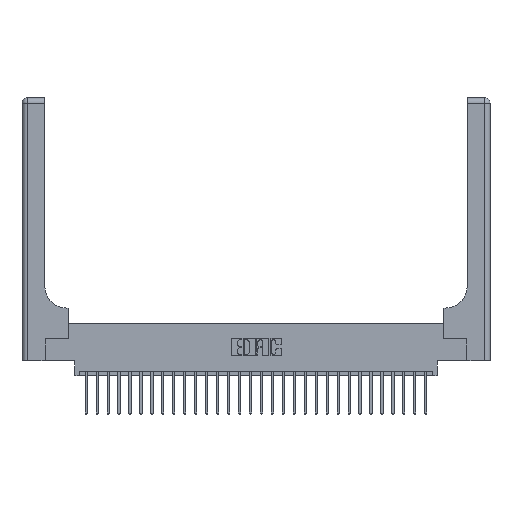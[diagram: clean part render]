
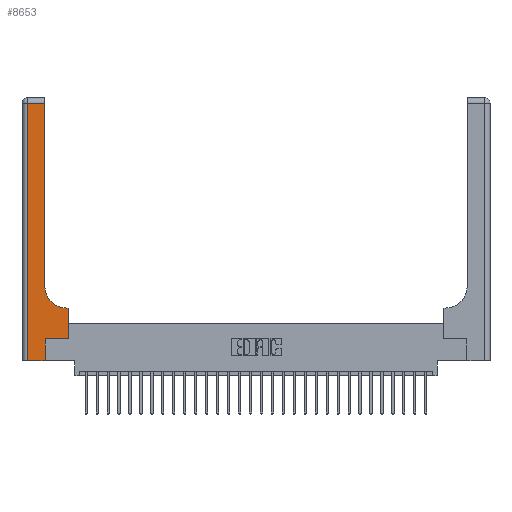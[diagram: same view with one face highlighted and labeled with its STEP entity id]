
A CAD part, top view. The second image highlights one B-rep face of the part: STEP entity #8653.
In plain terms, the highlighted planar face has unit normal (0, 0, 1).
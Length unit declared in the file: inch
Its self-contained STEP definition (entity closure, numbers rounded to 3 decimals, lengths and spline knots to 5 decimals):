
#243 = CARTESIAN_POINT ( 'NONE',  ( 0., 0., 0.37 ) ) ;
#2064 = VERTEX_POINT ( 'NONE', #19574 ) ;
#2099 = AXIS2_PLACEMENT_3D ( 'NONE', #23256, #10448, #25402 ) ;
#2349 = DIRECTION ( 'NONE',  ( 1., 0., 0. ) ) ;
#2496 = VERTEX_POINT ( 'NONE', #19162 ) ;
#2763 = EDGE_CURVE ( 'NONE', #27196, #2496, #19982, .T. ) ;
#3000 = VERTEX_POINT ( 'NONE', #27506 ) ;
#3001 = CIRCLE ( 'NONE', #2099, 0.25 ) ;
#3033 = LINE ( 'NONE', #22106, #20047 ) ;
#3495 = CARTESIAN_POINT ( 'NONE',  ( 0., 2.94, 0.37 ) ) ;
#3851 = VECTOR ( 'NONE', #6692, 39.37008 ) ;
#4194 = EDGE_CURVE ( 'NONE', #2064, #27196, #26249, .T. ) ;
#4537 = CARTESIAN_POINT ( 'NONE',  ( 0.528, 0.25, 0.37 ) ) ;
#4906 = CARTESIAN_POINT ( 'NONE',  ( 0.06, 2.94, 0.37 ) ) ;
#5364 = ORIENTED_EDGE ( 'NONE', *, *, #2763, .T. ) ;
#6692 = DIRECTION ( 'NONE',  ( 0., 1., 0. ) ) ;
#7667 = DIRECTION ( 'NONE',  ( 0., -1., 0. ) ) ;
#7842 = CARTESIAN_POINT ( 'NONE',  ( 0.26, 0.85, 0.37 ) ) ;
#8341 = VECTOR ( 'NONE', #26513, 39.37008 ) ;
#8450 = AXIS2_PLACEMENT_3D ( 'NONE', #23636, #10837, #25774 ) ;
#8653 = ADVANCED_FACE ( 'NONE', ( #12658 ), #19362, .F. ) ;
#8749 = CARTESIAN_POINT ( 'NONE',  ( 0.51, 0.6, 0.37 ) ) ;
#8845 = VECTOR ( 'NONE', #15403, 39.37008 ) ;
#8853 = EDGE_CURVE ( 'NONE', #15302, #2064, #12974, .T. ) ;
#9076 = EDGE_LOOP ( 'NONE', ( #20608, #18753, #5364, #17082, #13616, #17212, #23130, #24506, #11147 ) ) ;
#9477 = VERTEX_POINT ( 'NONE', #11938 ) ;
#10448 = DIRECTION ( 'NONE',  ( 0., 0., -1. ) ) ;
#10837 = DIRECTION ( 'NONE',  ( 0., 0., -1. ) ) ;
#11147 = ORIENTED_EDGE ( 'NONE', *, *, #22195, .T. ) ;
#11436 = DIRECTION ( 'NONE',  ( 0., 1., 0. ) ) ;
#11895 = VERTEX_POINT ( 'NONE', #8749 ) ;
#11938 = CARTESIAN_POINT ( 'NONE',  ( 0.265, 0., 0.37 ) ) ;
#11957 = CARTESIAN_POINT ( 'NONE',  ( 0.06, 3., 0.37 ) ) ;
#12104 = EDGE_CURVE ( 'NONE', #9477, #17315, #3033, .T. ) ;
#12658 = FACE_OUTER_BOUND ( 'NONE', #9076, .T. ) ;
#12816 = EDGE_CURVE ( 'NONE', #3000, #11895, #14698, .T. ) ;
#12974 = LINE ( 'NONE', #13944, #18031 ) ;
#13616 = ORIENTED_EDGE ( 'NONE', *, *, #12104, .T. ) ;
#13944 = CARTESIAN_POINT ( 'NONE',  ( 0.26, 3., 0.37 ) ) ;
#14698 = LINE ( 'NONE', #20083, #8341 ) ;
#15302 = VERTEX_POINT ( 'NONE', #7842 ) ;
#15403 = DIRECTION ( 'NONE',  ( 1., 0., 0. ) ) ;
#15508 = EDGE_CURVE ( 'NONE', #15823, #3000, #20893, .T. ) ;
#15557 = EDGE_CURVE ( 'NONE', #17315, #15823, #25217, .T. ) ;
#15823 = VERTEX_POINT ( 'NONE', #24795 ) ;
#17082 = ORIENTED_EDGE ( 'NONE', *, *, #21582, .T. ) ;
#17212 = ORIENTED_EDGE ( 'NONE', *, *, #15557, .T. ) ;
#17315 = VERTEX_POINT ( 'NONE', #26492 ) ;
#18031 = VECTOR ( 'NONE', #22429, 39.37008 ) ;
#18363 = DIRECTION ( 'NONE',  ( -1., 0., 0. ) ) ;
#18753 = ORIENTED_EDGE ( 'NONE', *, *, #4194, .T. ) ;
#19162 = CARTESIAN_POINT ( 'NONE',  ( 0.06, 0., 0.37 ) ) ;
#19362 = PLANE ( 'NONE',  #8450 ) ;
#19574 = CARTESIAN_POINT ( 'NONE',  ( 0.26, 2.94, 0.37 ) ) ;
#19906 = VECTOR ( 'NONE', #18363, 39.37008 ) ;
#19982 = LINE ( 'NONE', #11957, #25656 ) ;
#20047 = VECTOR ( 'NONE', #11436, 39.37008 ) ;
#20083 = CARTESIAN_POINT ( 'NONE',  ( 0.26, 0.6, 0.37 ) ) ;
#20608 = ORIENTED_EDGE ( 'NONE', *, *, #8853, .T. ) ;
#20893 = LINE ( 'NONE', #4537, #3851 ) ;
#21582 = EDGE_CURVE ( 'NONE', #2496, #9477, #22514, .T. ) ;
#21730 = CARTESIAN_POINT ( 'NONE',  ( 0.265, 0.25, 0.37 ) ) ;
#21845 = VECTOR ( 'NONE', #2349, 39.37008 ) ;
#22106 = CARTESIAN_POINT ( 'NONE',  ( 0.265, 0., 0.37 ) ) ;
#22195 = EDGE_CURVE ( 'NONE', #11895, #15302, #3001, .T. ) ;
#22429 = DIRECTION ( 'NONE',  ( 0., 1., 0. ) ) ;
#22514 = LINE ( 'NONE', #243, #21845 ) ;
#23130 = ORIENTED_EDGE ( 'NONE', *, *, #15508, .T. ) ;
#23256 = CARTESIAN_POINT ( 'NONE',  ( 0.51, 0.85, 0.37 ) ) ;
#23636 = CARTESIAN_POINT ( 'NONE',  ( 0., 3., 0.37 ) ) ;
#24506 = ORIENTED_EDGE ( 'NONE', *, *, #12816, .T. ) ;
#24795 = CARTESIAN_POINT ( 'NONE',  ( 0.528, 0.25, 0.37 ) ) ;
#25217 = LINE ( 'NONE', #21730, #8845 ) ;
#25402 = DIRECTION ( 'NONE',  ( 1., 0., 0. ) ) ;
#25656 = VECTOR ( 'NONE', #7667, 39.37008 ) ;
#25774 = DIRECTION ( 'NONE',  ( -1., 0., 0. ) ) ;
#26249 = LINE ( 'NONE', #3495, #19906 ) ;
#26492 = CARTESIAN_POINT ( 'NONE',  ( 0.265, 0.25, 0.37 ) ) ;
#26513 = DIRECTION ( 'NONE',  ( -1., 0., 0. ) ) ;
#27196 = VERTEX_POINT ( 'NONE', #4906 ) ;
#27506 = CARTESIAN_POINT ( 'NONE',  ( 0.528, 0.6, 0.37 ) ) ;
